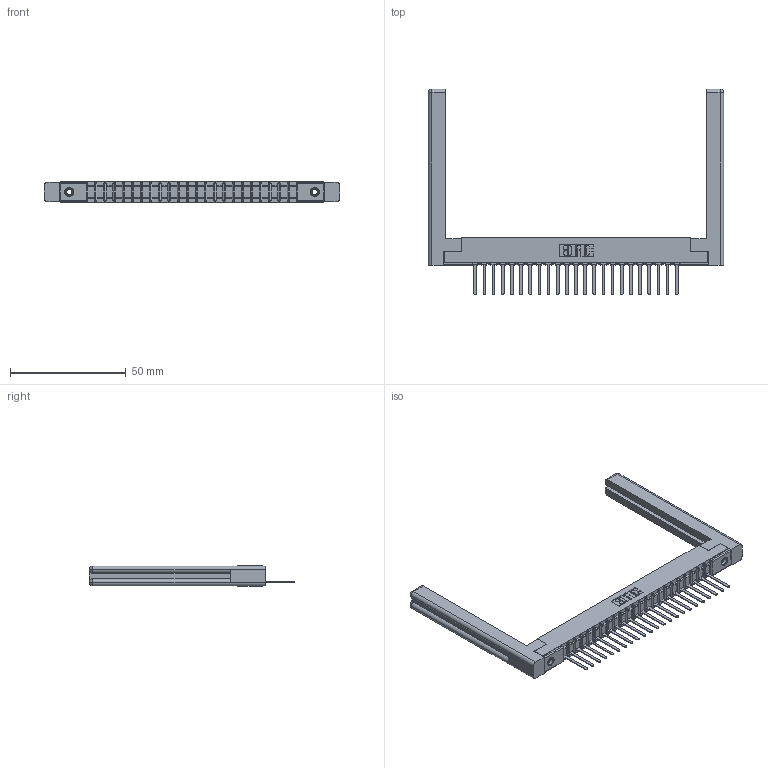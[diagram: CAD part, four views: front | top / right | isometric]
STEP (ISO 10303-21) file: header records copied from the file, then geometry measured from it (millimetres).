
FILE_DESCRIPTION (( 'STEP AP203' ), '1' );
FILE_NAME ('307-023-441-158.STEP', '2020-09-27T09:11:35', ( '' ), ( '' ), 'SwSTEP 2.0', 'SolidWorks 2020', '' );
FILE_SCHEMA (( 'CONFIG_CONTROL_DESIGN' ));
Length unit declared in the file: inch
Products named in the file (5): 307 Part_.156 Dia Mounting Holes; 345-250-001_345-250-001-102; 307-290-002_541; 307-023-441-158; 307-220-058
Assembly tree (28 placements, depth 2):
  307-023-441-158
    307 Part_.156 Dia Mounting Holes
    307-290-002_541  x23
    307-220-058  x2
    345-250-001_345-250-001-102  x2
Bounding box: 127.76 x 88.9 x 8.71 mm (x, y, z)
Volume: 16178.4 mm3; surface area: 20932 mm2
Topology: 28 solids, 28 shells, 1986 faces, 6013 edges, 3930 vertices
Faces by surface type: plane 1189, cylinder 725, sphere 48, torus 12, cone 12
Entity records: 25411 total; most frequent: CARTESIAN_POINT 4291, ORIENTED_EDGE 4220, DIRECTION 4138, EDGE_CURVE 2110, VECTOR 1604, LINE 1604, VERTEX_POINT 1366, AXIS2_PLACEMENT_3D 1267
